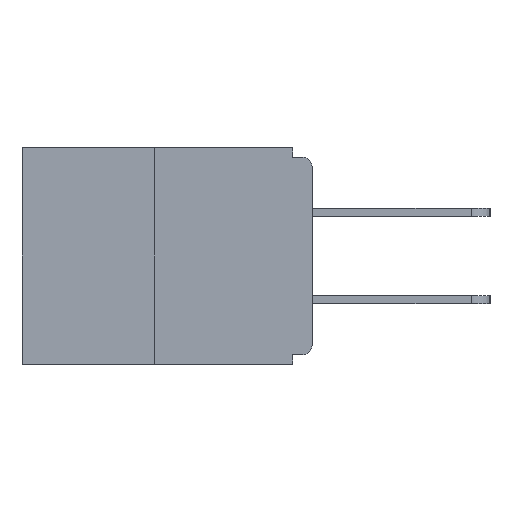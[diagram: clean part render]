
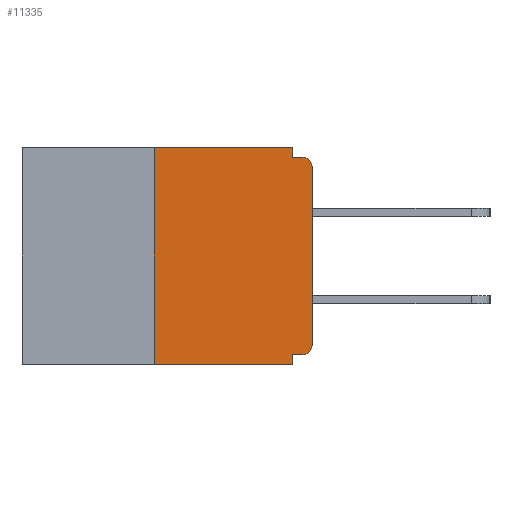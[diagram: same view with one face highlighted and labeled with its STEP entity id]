
A CAD part, left-side view. The second image highlights one B-rep face of the part: STEP entity #11335.
In plain terms, the highlighted planar face has unit normal (-1, 0, 0).
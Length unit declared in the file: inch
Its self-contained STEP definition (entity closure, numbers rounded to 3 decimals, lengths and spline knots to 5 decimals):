
#543 = CARTESIAN_POINT ( 'NONE',  ( 0., 0.031, -0.343 ) ) ;
#779 = EDGE_LOOP ( 'NONE', ( #9198, #15358, #10668, #950, #16461, #10445, #21132, #3525, #2781, #4316 ) ) ;
#950 = ORIENTED_EDGE ( 'NONE', *, *, #3157, .F. ) ;
#1045 = VECTOR ( 'NONE', #2318, 39.37008 ) ;
#1094 = VERTEX_POINT ( 'NONE', #12176 ) ;
#1202 = CARTESIAN_POINT ( 'NONE',  ( 0., 0., -0.313 ) ) ;
#1274 = LINE ( 'NONE', #15794, #14816 ) ;
#1305 = LINE ( 'NONE', #12694, #1045 ) ;
#1474 = VERTEX_POINT ( 'NONE', #14623 ) ;
#1747 = VECTOR ( 'NONE', #4814, 39.37008 ) ;
#1864 = EDGE_CURVE ( 'NONE', #6863, #9128, #13288, .T. ) ;
#2088 = DIRECTION ( 'NONE',  ( -1., 0., 0. ) ) ;
#2112 = DIRECTION ( 'NONE',  ( 0., 0., -1. ) ) ;
#2201 = LINE ( 'NONE', #15253, #2458 ) ;
#2318 = DIRECTION ( 'NONE',  ( 0., 0., -1. ) ) ;
#2434 = CARTESIAN_POINT ( 'NONE',  ( 0., 0.25, -0.343 ) ) ;
#2458 = VECTOR ( 'NONE', #8343, 39.37008 ) ;
#2485 = DIRECTION ( 'NONE',  ( 0., 0., -1. ) ) ;
#2739 = AXIS2_PLACEMENT_3D ( 'NONE', #7379, #14219, #2112 ) ;
#2757 = VECTOR ( 'NONE', #6962, 39.37008 ) ;
#2781 = ORIENTED_EDGE ( 'NONE', *, *, #1864, .F. ) ;
#3056 = CARTESIAN_POINT ( 'NONE',  ( 0., 0., 0. ) ) ;
#3074 = VECTOR ( 'NONE', #13583, 39.37008 ) ;
#3157 = EDGE_CURVE ( 'NONE', #1094, #20802, #11923, .T. ) ;
#3260 = CIRCLE ( 'NONE', #7957, 0.015 ) ;
#3492 = CARTESIAN_POINT ( 'NONE',  ( 0., 0.46, -0.343 ) ) ;
#3525 = ORIENTED_EDGE ( 'NONE', *, *, #10917, .T. ) ;
#4039 = CARTESIAN_POINT ( 'NONE',  ( 0., 0.031, -0.343 ) ) ;
#4316 = ORIENTED_EDGE ( 'NONE', *, *, #12351, .F. ) ;
#4814 = DIRECTION ( 'NONE',  ( 0., 0., 1. ) ) ;
#6233 = DIRECTION ( 'NONE',  ( 0., 0., -1. ) ) ;
#6452 = EDGE_CURVE ( 'NONE', #1474, #17909, #1274, .T. ) ;
#6863 = VERTEX_POINT ( 'NONE', #19842 ) ;
#6962 = DIRECTION ( 'NONE',  ( 0., -1., 0. ) ) ;
#7153 = LINE ( 'NONE', #11833, #1747 ) ;
#7351 = LINE ( 'NONE', #3492, #2757 ) ;
#7379 = CARTESIAN_POINT ( 'NONE',  ( 0., 0.46, 0. ) ) ;
#7456 = PLANE ( 'NONE',  #2739 ) ;
#7528 = CARTESIAN_POINT ( 'NONE',  ( 0., 0.015, -0.328 ) ) ;
#7671 = EDGE_CURVE ( 'NONE', #16599, #1474, #7153, .T. ) ;
#7957 = AXIS2_PLACEMENT_3D ( 'NONE', #19938, #21678, #6233 ) ;
#8343 = DIRECTION ( 'NONE',  ( 0., 1., 0. ) ) ;
#8772 = LINE ( 'NONE', #3056, #3074 ) ;
#9128 = VERTEX_POINT ( 'NONE', #18786 ) ;
#9198 = ORIENTED_EDGE ( 'NONE', *, *, #6452, .F. ) ;
#10186 = EDGE_CURVE ( 'NONE', #16599, #20802, #7351, .T. ) ;
#10445 = ORIENTED_EDGE ( 'NONE', *, *, #14770, .T. ) ;
#10668 = ORIENTED_EDGE ( 'NONE', *, *, #10186, .T. ) ;
#10917 = EDGE_CURVE ( 'NONE', #17772, #9128, #3260, .T. ) ;
#11330 = CARTESIAN_POINT ( 'NONE',  ( 0., 0., -0.015 ) ) ;
#11335 = ADVANCED_FACE ( 'NONE', ( #19499 ), #7456, .F. ) ;
#11392 = VECTOR ( 'NONE', #21400, 39.37008 ) ;
#11833 = CARTESIAN_POINT ( 'NONE',  ( 0., 0.25, 0. ) ) ;
#11923 = LINE ( 'NONE', #543, #12484 ) ;
#12176 = CARTESIAN_POINT ( 'NONE',  ( 0., 0.031, -0.328 ) ) ;
#12333 = CARTESIAN_POINT ( 'NONE',  ( 0., 0.031, 0. ) ) ;
#12351 = EDGE_CURVE ( 'NONE', #17909, #6863, #1305, .T. ) ;
#12484 = VECTOR ( 'NONE', #2485, 39.37008 ) ;
#12694 = CARTESIAN_POINT ( 'NONE',  ( 0., 0.031, 0. ) ) ;
#13288 = LINE ( 'NONE', #11330, #11392 ) ;
#13583 = DIRECTION ( 'NONE',  ( 0., 0., 1. ) ) ;
#14195 = DIRECTION ( 'NONE',  ( 0., 0., -1. ) ) ;
#14219 = DIRECTION ( 'NONE',  ( 1., 0., 0. ) ) ;
#14265 = AXIS2_PLACEMENT_3D ( 'NONE', #19259, #2088, #14195 ) ;
#14378 = EDGE_CURVE ( 'NONE', #15736, #17772, #8772, .T. ) ;
#14623 = CARTESIAN_POINT ( 'NONE',  ( 0., 0.25, 0. ) ) ;
#14770 = EDGE_CURVE ( 'NONE', #17123, #15736, #16117, .T. ) ;
#14816 = VECTOR ( 'NONE', #22430, 39.37008 ) ;
#15253 = CARTESIAN_POINT ( 'NONE',  ( 0., 0., -0.328 ) ) ;
#15358 = ORIENTED_EDGE ( 'NONE', *, *, #7671, .F. ) ;
#15736 = VERTEX_POINT ( 'NONE', #1202 ) ;
#15794 = CARTESIAN_POINT ( 'NONE',  ( 0., 0.46, 0. ) ) ;
#16117 = CIRCLE ( 'NONE', #14265, 0.015 ) ;
#16461 = ORIENTED_EDGE ( 'NONE', *, *, #21939, .F. ) ;
#16599 = VERTEX_POINT ( 'NONE', #2434 ) ;
#17123 = VERTEX_POINT ( 'NONE', #7528 ) ;
#17772 = VERTEX_POINT ( 'NONE', #18462 ) ;
#17909 = VERTEX_POINT ( 'NONE', #12333 ) ;
#18462 = CARTESIAN_POINT ( 'NONE',  ( 0., 0., -0.03 ) ) ;
#18786 = CARTESIAN_POINT ( 'NONE',  ( 0., 0.015, -0.015 ) ) ;
#19259 = CARTESIAN_POINT ( 'NONE',  ( 0., 0.015, -0.313 ) ) ;
#19499 = FACE_OUTER_BOUND ( 'NONE', #779, .T. ) ;
#19842 = CARTESIAN_POINT ( 'NONE',  ( 0., 0.031, -0.015 ) ) ;
#19938 = CARTESIAN_POINT ( 'NONE',  ( 0., 0.015, -0.03 ) ) ;
#20802 = VERTEX_POINT ( 'NONE', #4039 ) ;
#21132 = ORIENTED_EDGE ( 'NONE', *, *, #14378, .T. ) ;
#21400 = DIRECTION ( 'NONE',  ( 0., -1., 0. ) ) ;
#21678 = DIRECTION ( 'NONE',  ( -1., 0., 0. ) ) ;
#21939 = EDGE_CURVE ( 'NONE', #17123, #1094, #2201, .T. ) ;
#22430 = DIRECTION ( 'NONE',  ( 0., -1., 0. ) ) ;
